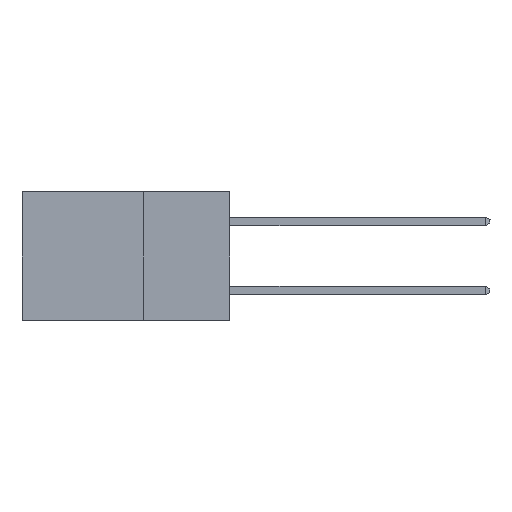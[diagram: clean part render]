
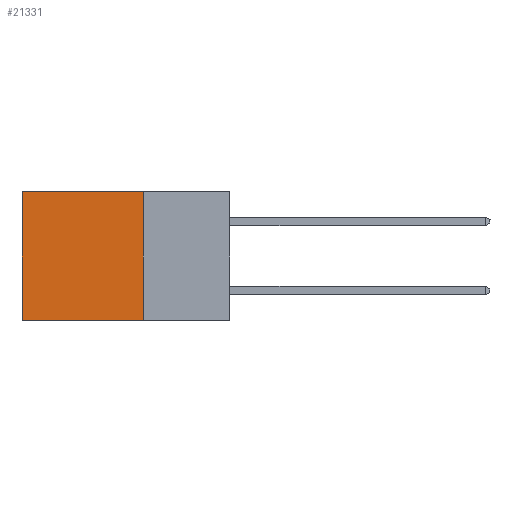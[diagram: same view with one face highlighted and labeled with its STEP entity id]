
A CAD part, left-side view. The second image highlights one B-rep face of the part: STEP entity #21331.
In plain terms, the highlighted planar face has unit normal (-1, 0, 0).
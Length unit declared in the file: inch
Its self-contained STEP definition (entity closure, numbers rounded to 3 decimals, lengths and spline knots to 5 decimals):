
#1537 = LINE ( 'NONE', #8771, #22273 ) ;
#1742 = EDGE_LOOP ( 'NONE', ( #16569, #10019, #10068, #3257 ) ) ;
#2031 = LINE ( 'NONE', #16666, #20714 ) ;
#2841 = LINE ( 'NONE', #10095, #10055 ) ;
#3257 = ORIENTED_EDGE ( 'NONE', *, *, #17640, .T. ) ;
#5078 = CARTESIAN_POINT ( 'NONE',  ( 0.2615, 0.25, -0.37 ) ) ;
#6548 = DIRECTION ( 'NONE',  ( 0., 1., 0. ) ) ;
#8305 = PLANE ( 'NONE',  #19039 ) ;
#8362 = EDGE_CURVE ( 'NONE', #9848, #18003, #1537, .T. ) ;
#8584 = LINE ( 'NONE', #11707, #13765 ) ;
#8771 = CARTESIAN_POINT ( 'NONE',  ( 0.2615, 0.6, -0.37 ) ) ;
#9848 = VERTEX_POINT ( 'NONE', #10182 ) ;
#10019 = ORIENTED_EDGE ( 'NONE', *, *, #15262, .F. ) ;
#10055 = VECTOR ( 'NONE', #11996, 39.37008 ) ;
#10068 = ORIENTED_EDGE ( 'NONE', *, *, #14328, .F. ) ;
#10095 = CARTESIAN_POINT ( 'NONE',  ( 0.2615, 0.25, 0. ) ) ;
#10182 = CARTESIAN_POINT ( 'NONE',  ( 0.2615, 0.6, 0. ) ) ;
#11324 = CARTESIAN_POINT ( 'NONE',  ( 0.2615, 0.6, -0.37 ) ) ;
#11707 = CARTESIAN_POINT ( 'NONE',  ( 0.2615, 0.25, -0.37 ) ) ;
#11996 = DIRECTION ( 'NONE',  ( 0., 1., 0. ) ) ;
#12025 = CARTESIAN_POINT ( 'NONE',  ( 0.2615, 0.25, -0.37 ) ) ;
#12086 = VERTEX_POINT ( 'NONE', #12025 ) ;
#13765 = VECTOR ( 'NONE', #6548, 39.37008 ) ;
#13910 = DIRECTION ( 'NONE',  ( 1., 0., 0. ) ) ;
#14328 = EDGE_CURVE ( 'NONE', #14837, #12086, #2031, .T. ) ;
#14837 = VERTEX_POINT ( 'NONE', #16729 ) ;
#15262 = EDGE_CURVE ( 'NONE', #12086, #18003, #8584, .T. ) ;
#16040 = DIRECTION ( 'NONE',  ( 0., 0., -1. ) ) ;
#16569 = ORIENTED_EDGE ( 'NONE', *, *, #8362, .T. ) ;
#16666 = CARTESIAN_POINT ( 'NONE',  ( 0.2615, 0.25, -0.37 ) ) ;
#16729 = CARTESIAN_POINT ( 'NONE',  ( 0.2615, 0.25, 0. ) ) ;
#17598 = FACE_OUTER_BOUND ( 'NONE', #1742, .T. ) ;
#17640 = EDGE_CURVE ( 'NONE', #14837, #9848, #2841, .T. ) ;
#18003 = VERTEX_POINT ( 'NONE', #11324 ) ;
#19039 = AXIS2_PLACEMENT_3D ( 'NONE', #5078, #13910, #21105 ) ;
#20071 = DIRECTION ( 'NONE',  ( 0., 0., -1. ) ) ;
#20714 = VECTOR ( 'NONE', #20071, 39.37008 ) ;
#21105 = DIRECTION ( 'NONE',  ( 0., 0., -1. ) ) ;
#21331 = ADVANCED_FACE ( 'NONE', ( #17598 ), #8305, .F. ) ;
#22273 = VECTOR ( 'NONE', #16040, 39.37008 ) ;
